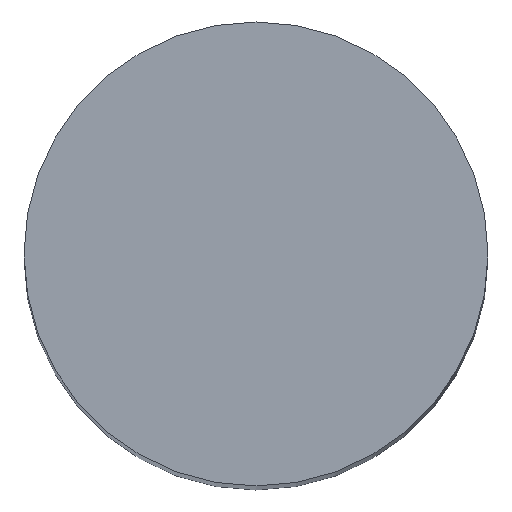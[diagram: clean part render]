
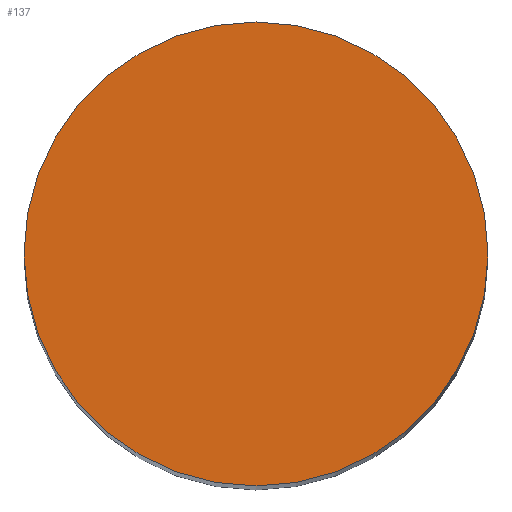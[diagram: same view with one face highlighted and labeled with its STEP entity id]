
A CAD part, top view. The second image highlights one B-rep face of the part: STEP entity #137.
In plain terms, the highlighted planar face has unit normal (0, 0, 1).
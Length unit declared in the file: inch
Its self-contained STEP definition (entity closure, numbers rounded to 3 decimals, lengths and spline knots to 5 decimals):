
#3 = DIRECTION ( 'NONE',  ( 0., 0., 1. ) ) ;
#7 = EDGE_LOOP ( 'NONE', ( #43, #67 ) ) ;
#11 = CIRCLE ( 'NONE', #105, 0.1 ) ;
#14 = CARTESIAN_POINT ( 'NONE',  ( 0., 0., 1. ) ) ;
#17 = AXIS2_PLACEMENT_3D ( 'NONE', #32, #3, #55 ) ;
#30 = AXIS2_PLACEMENT_3D ( 'NONE', #14, #84, #44 ) ;
#32 = CARTESIAN_POINT ( 'NONE',  ( 0., 0., 1. ) ) ;
#42 = DIRECTION ( 'NONE',  ( 0., 0., 1. ) ) ;
#43 = ORIENTED_EDGE ( 'NONE', *, *, #78, .T. ) ;
#44 = DIRECTION ( 'NONE',  ( 1., 0., 0. ) ) ;
#45 = CARTESIAN_POINT ( 'NONE',  ( 0., 0., 1. ) ) ;
#54 = CARTESIAN_POINT ( 'NONE',  ( 0.1, 0., 1. ) ) ;
#55 = DIRECTION ( 'NONE',  ( 1., 0., 0. ) ) ;
#63 = FACE_OUTER_BOUND ( 'NONE', #7, .T. ) ;
#67 = ORIENTED_EDGE ( 'NONE', *, *, #106, .T. ) ;
#68 = CARTESIAN_POINT ( 'NONE',  ( -0.1, 0., 1. ) ) ;
#78 = EDGE_CURVE ( 'NONE', #136, #92, #143, .T. ) ;
#83 = DIRECTION ( 'NONE',  ( 1., 0., 0. ) ) ;
#84 = DIRECTION ( 'NONE',  ( 0., 0., 1. ) ) ;
#92 = VERTEX_POINT ( 'NONE', #54 ) ;
#105 = AXIS2_PLACEMENT_3D ( 'NONE', #45, #42, #83 ) ;
#106 = EDGE_CURVE ( 'NONE', #92, #136, #11, .T. ) ;
#108 = PLANE ( 'NONE',  #17 ) ;
#136 = VERTEX_POINT ( 'NONE', #68 ) ;
#137 = ADVANCED_FACE ( 'NONE', ( #63 ), #108, .T. ) ;
#143 = CIRCLE ( 'NONE', #30, 0.1 ) ;
